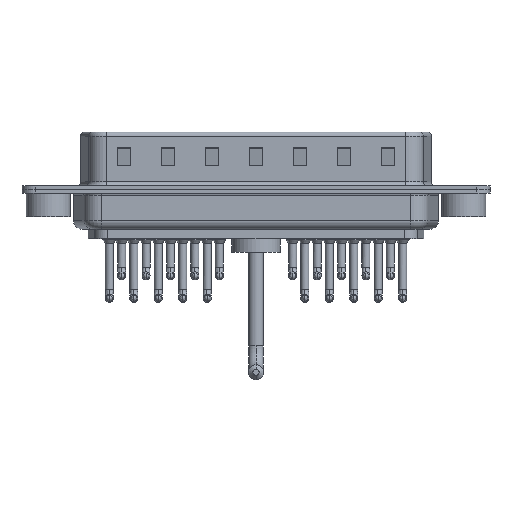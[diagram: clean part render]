
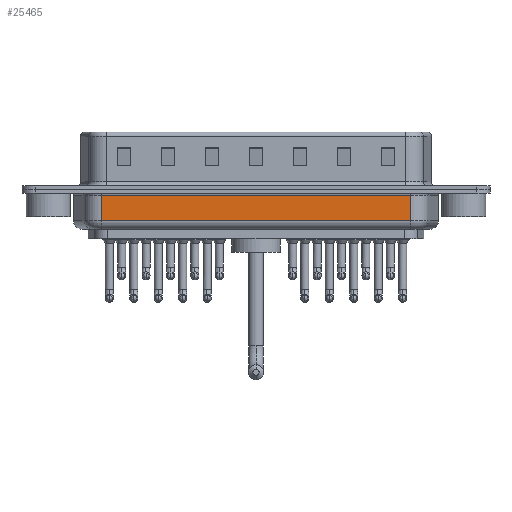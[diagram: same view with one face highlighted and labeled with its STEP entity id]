
A CAD part, front view. The second image highlights one B-rep face of the part: STEP entity #25465.
In plain terms, the highlighted planar face has unit normal (0, -1, 0).
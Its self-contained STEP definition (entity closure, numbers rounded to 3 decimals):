
#210 = CARTESIAN_POINT ( 'NONE',  ( 41.044, -5.35, -3.5 ) ) ;
#610 = VERTEX_POINT ( 'NONE', #210 ) ;
#1197 = ORIENTED_EDGE ( 'NONE', *, *, #18272, .T. ) ;
#1992 = ORIENTED_EDGE ( 'NONE', *, *, #11929, .T. ) ;
#2029 = DIRECTION ( 'NONE',  ( 1., 0., 0. ) ) ;
#2378 = CARTESIAN_POINT ( 'NONE',  ( 6.006, -5.35, -4.5 ) ) ;
#2441 = LINE ( 'NONE', #10430, #13373 ) ;
#3397 = EDGE_LOOP ( 'NONE', ( #12780, #23739, #1197, #1992 ) ) ;
#4346 = PLANE ( 'NONE',  #25616 ) ;
#5393 = DIRECTION ( 'NONE',  ( -1., 0., 0. ) ) ;
#6097 = VECTOR ( 'NONE', #13067, 1000. ) ;
#7149 = VECTOR ( 'NONE', #5393, 1000. ) ;
#7372 = CARTESIAN_POINT ( 'NONE',  ( 6.006, -5.35, -0.65 ) ) ;
#8265 = VERTEX_POINT ( 'NONE', #24189 ) ;
#8788 = VERTEX_POINT ( 'NONE', #14130 ) ;
#10430 = CARTESIAN_POINT ( 'NONE',  ( 6.006, -5.35, -4.5 ) ) ;
#11929 = EDGE_CURVE ( 'NONE', #22122, #8265, #19300, .T. ) ;
#12334 = CARTESIAN_POINT ( 'NONE',  ( 41.044, -5.35, -4.5 ) ) ;
#12780 = ORIENTED_EDGE ( 'NONE', *, *, #22279, .F. ) ;
#13067 = DIRECTION ( 'NONE',  ( 0., 0., 1. ) ) ;
#13373 = VECTOR ( 'NONE', #18418, 1000. ) ;
#14130 = CARTESIAN_POINT ( 'NONE',  ( 6.006, -5.35, -3.5 ) ) ;
#14432 = LINE ( 'NONE', #12334, #6097 ) ;
#18272 = EDGE_CURVE ( 'NONE', #610, #22122, #14432, .T. ) ;
#18418 = DIRECTION ( 'NONE',  ( 0., 0., 1. ) ) ;
#18490 = DIRECTION ( 'NONE',  ( 0., 1., 0. ) ) ;
#19300 = LINE ( 'NONE', #7372, #7149 ) ;
#19729 = CARTESIAN_POINT ( 'NONE',  ( 6.006, -5.35, -3.5 ) ) ;
#20516 = VECTOR ( 'NONE', #2029, 1000. ) ;
#22122 = VERTEX_POINT ( 'NONE', #24982 ) ;
#22279 = EDGE_CURVE ( 'NONE', #8788, #8265, #2441, .T. ) ;
#22305 = FACE_OUTER_BOUND ( 'NONE', #3397, .T. ) ;
#22436 = DIRECTION ( 'NONE',  ( 0., 0., 1. ) ) ;
#22576 = EDGE_CURVE ( 'NONE', #8788, #610, #23925, .T. ) ;
#23739 = ORIENTED_EDGE ( 'NONE', *, *, #22576, .T. ) ;
#23925 = LINE ( 'NONE', #19729, #20516 ) ;
#24189 = CARTESIAN_POINT ( 'NONE',  ( 6.006, -5.35, -0.65 ) ) ;
#24982 = CARTESIAN_POINT ( 'NONE',  ( 41.044, -5.35, -0.65 ) ) ;
#25465 = ADVANCED_FACE ( 'NONE', ( #22305 ), #4346, .F. ) ;
#25616 = AXIS2_PLACEMENT_3D ( 'NONE', #2378, #18490, #22436 ) ;
